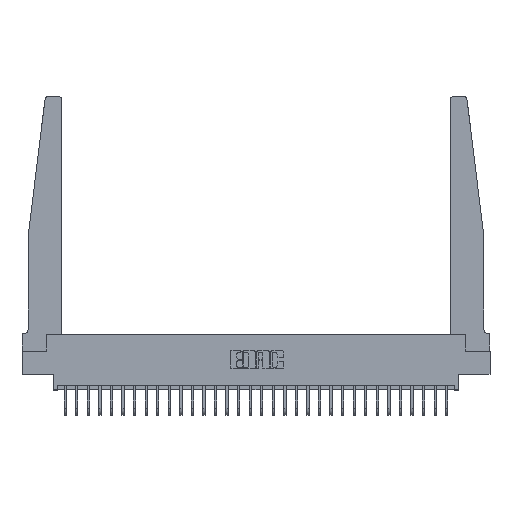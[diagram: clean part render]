
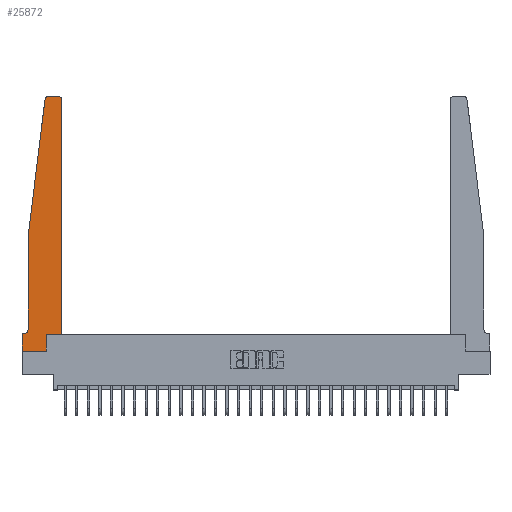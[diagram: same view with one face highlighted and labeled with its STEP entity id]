
A CAD part, top view. The second image highlights one B-rep face of the part: STEP entity #25872.
In plain terms, the highlighted planar face has unit normal (0, 0, 1).
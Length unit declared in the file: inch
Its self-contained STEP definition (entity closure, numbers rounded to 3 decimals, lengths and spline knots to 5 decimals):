
#202 = EDGE_CURVE ( 'NONE', #3517, #4428, #2858, .T. ) ;
#236 = AXIS2_PLACEMENT_3D ( 'NONE', #23653, #11117, #25749 ) ;
#385 = LINE ( 'NONE', #25950, #16533 ) ;
#737 = PLANE ( 'NONE',  #3675 ) ;
#984 = VERTEX_POINT ( 'NONE', #1517 ) ;
#1458 = EDGE_CURVE ( 'NONE', #24865, #11048, #17905, .T. ) ;
#1476 = ORIENTED_EDGE ( 'NONE', *, *, #18724, .T. ) ;
#1517 = CARTESIAN_POINT ( 'NONE',  ( 0.395, 2.75, 0.37 ) ) ;
#1602 = CARTESIAN_POINT ( 'NONE',  ( 0., 0., 0.37 ) ) ;
#1694 = ORIENTED_EDGE ( 'NONE', *, *, #8246, .T. ) ;
#2197 = VECTOR ( 'NONE', #7533, 39.37008 ) ;
#2371 = DIRECTION ( 'NONE',  ( 1., 0., 0. ) ) ;
#2480 = LINE ( 'NONE', #26995, #14278 ) ;
#2668 = CARTESIAN_POINT ( 'NONE',  ( 0.065, 1.25, 0.37 ) ) ;
#2858 = LINE ( 'NONE', #16054, #2197 ) ;
#3030 = VERTEX_POINT ( 'NONE', #4614 ) ;
#3064 = CARTESIAN_POINT ( 'NONE',  ( 0.27653, 2.75, 0.37 ) ) ;
#3068 = ORIENTED_EDGE ( 'NONE', *, *, #202, .T. ) ;
#3286 = CARTESIAN_POINT ( 'NONE',  ( 0.065, 1.25, 0.37 ) ) ;
#3517 = VERTEX_POINT ( 'NONE', #15203 ) ;
#3675 = AXIS2_PLACEMENT_3D ( 'NONE', #17577, #5014, #19673 ) ;
#3936 = EDGE_CURVE ( 'NONE', #25004, #24865, #8726, .T. ) ;
#4331 = VECTOR ( 'NONE', #26123, 39.37008 ) ;
#4428 = VERTEX_POINT ( 'NONE', #3286 ) ;
#4562 = DIRECTION ( 'NONE',  ( 0., 0., 1. ) ) ;
#4614 = CARTESIAN_POINT ( 'NONE',  ( 0.015, 0.1875, 0.37 ) ) ;
#4989 = EDGE_LOOP ( 'NONE', ( #1694, #9234, #3068, #1476, #12937, #21291, #25565, #26475, #20586, #14266, #13524, #8286 ) ) ;
#5014 = DIRECTION ( 'NONE',  ( 0., 0., 1. ) ) ;
#5587 = CARTESIAN_POINT ( 'NONE',  ( 0.2605, 0., 0.37 ) ) ;
#5908 = CARTESIAN_POINT ( 'NONE',  ( 0.015, 0.2375, 0.37 ) ) ;
#6097 = AXIS2_PLACEMENT_3D ( 'NONE', #17130, #4562, #19234 ) ;
#6887 = VERTEX_POINT ( 'NONE', #3064 ) ;
#6914 = EDGE_CURVE ( 'NONE', #13854, #25004, #7936, .T. ) ;
#7533 = DIRECTION ( 'NONE',  ( -0.122, -0.992, 0. ) ) ;
#7851 = AXIS2_PLACEMENT_3D ( 'NONE', #5908, #20555, #8011 ) ;
#7936 = LINE ( 'NONE', #11473, #4331 ) ;
#8011 = DIRECTION ( 'NONE',  ( -1., 0., 0. ) ) ;
#8246 = EDGE_CURVE ( 'NONE', #984, #6887, #25530, .T. ) ;
#8286 = ORIENTED_EDGE ( 'NONE', *, *, #12758, .T. ) ;
#8726 = LINE ( 'NONE', #17132, #19227 ) ;
#8829 = VECTOR ( 'NONE', #17255, 39.37008 ) ;
#9234 = ORIENTED_EDGE ( 'NONE', *, *, #12041, .T. ) ;
#10289 = CARTESIAN_POINT ( 'NONE',  ( 0.2605, 0.18, 0.37 ) ) ;
#10714 = CIRCLE ( 'NONE', #236, 0.03 ) ;
#10925 = CARTESIAN_POINT ( 'NONE',  ( 0.25, 2.75, 0.37 ) ) ;
#11048 = VERTEX_POINT ( 'NONE', #17717 ) ;
#11117 = DIRECTION ( 'NONE',  ( 0., 0., 1. ) ) ;
#11409 = DIRECTION ( 'NONE',  ( 0., 1., 0. ) ) ;
#11413 = VERTEX_POINT ( 'NONE', #12524 ) ;
#11473 = CARTESIAN_POINT ( 'NONE',  ( 0.2605, 0.18, 0.37 ) ) ;
#11853 = VERTEX_POINT ( 'NONE', #1602 ) ;
#12041 = EDGE_CURVE ( 'NONE', #6887, #3517, #22228, .T. ) ;
#12279 = VECTOR ( 'NONE', #11409, 39.37008 ) ;
#12524 = CARTESIAN_POINT ( 'NONE',  ( 0.065, 0.2375, 0.37 ) ) ;
#12758 = EDGE_CURVE ( 'NONE', #11048, #984, #10714, .T. ) ;
#12851 = VECTOR ( 'NONE', #2371, 39.37008 ) ;
#12937 = ORIENTED_EDGE ( 'NONE', *, *, #24080, .T. ) ;
#13348 = EDGE_CURVE ( 'NONE', #21468, #11853, #2480, .T. ) ;
#13512 = LINE ( 'NONE', #17061, #12851 ) ;
#13524 = ORIENTED_EDGE ( 'NONE', *, *, #1458, .T. ) ;
#13854 = VERTEX_POINT ( 'NONE', #5587 ) ;
#14266 = ORIENTED_EDGE ( 'NONE', *, *, #3936, .T. ) ;
#14278 = VECTOR ( 'NONE', #14477, 39.37008 ) ;
#14477 = DIRECTION ( 'NONE',  ( 0., -1., 0. ) ) ;
#14757 = VECTOR ( 'NONE', #17362, 39.37008 ) ;
#15203 = CARTESIAN_POINT ( 'NONE',  ( 0.24675, 2.72367, 0.37 ) ) ;
#15535 = CARTESIAN_POINT ( 'NONE',  ( 0.425, 0.18, 0.37 ) ) ;
#15771 = CIRCLE ( 'NONE', #7851, 0.05 ) ;
#15826 = CARTESIAN_POINT ( 'NONE',  ( 0., 0.1875, 0.37 ) ) ;
#16054 = CARTESIAN_POINT ( 'NONE',  ( 0.065, 1.25, 0.37 ) ) ;
#16533 = VECTOR ( 'NONE', #23948, 39.37008 ) ;
#17049 = EDGE_CURVE ( 'NONE', #3030, #21468, #385, .T. ) ;
#17061 = CARTESIAN_POINT ( 'NONE',  ( 0., 0., 0.37 ) ) ;
#17130 = CARTESIAN_POINT ( 'NONE',  ( 0.27653, 2.72, 0.37 ) ) ;
#17132 = CARTESIAN_POINT ( 'NONE',  ( 0.425, 0.18, 0.37 ) ) ;
#17255 = DIRECTION ( 'NONE',  ( -1., 0., 0. ) ) ;
#17362 = DIRECTION ( 'NONE',  ( 0., -1., 0. ) ) ;
#17577 = CARTESIAN_POINT ( 'NONE',  ( 0., 0.1875, 0.37 ) ) ;
#17717 = CARTESIAN_POINT ( 'NONE',  ( 0.425, 2.72, 0.37 ) ) ;
#17905 = LINE ( 'NONE', #15535, #12279 ) ;
#18724 = EDGE_CURVE ( 'NONE', #4428, #11413, #20345, .T. ) ;
#19153 = DIRECTION ( 'NONE',  ( 1., 0., 0. ) ) ;
#19227 = VECTOR ( 'NONE', #19153, 39.37008 ) ;
#19234 = DIRECTION ( 'NONE',  ( 1., 0., 0. ) ) ;
#19673 = DIRECTION ( 'NONE',  ( 1., 0., 0. ) ) ;
#20345 = LINE ( 'NONE', #2668, #14757 ) ;
#20555 = DIRECTION ( 'NONE',  ( 0., 0., -1. ) ) ;
#20583 = FACE_OUTER_BOUND ( 'NONE', #4989, .T. ) ;
#20586 = ORIENTED_EDGE ( 'NONE', *, *, #6914, .T. ) ;
#21291 = ORIENTED_EDGE ( 'NONE', *, *, #17049, .T. ) ;
#21468 = VERTEX_POINT ( 'NONE', #15826 ) ;
#22228 = CIRCLE ( 'NONE', #6097, 0.03 ) ;
#22974 = EDGE_CURVE ( 'NONE', #11853, #13854, #13512, .T. ) ;
#23653 = CARTESIAN_POINT ( 'NONE',  ( 0.395, 2.72, 0.37 ) ) ;
#23948 = DIRECTION ( 'NONE',  ( -1., 0., 0. ) ) ;
#24080 = EDGE_CURVE ( 'NONE', #11413, #3030, #15771, .T. ) ;
#24458 = CARTESIAN_POINT ( 'NONE',  ( 0.425, 0.18, 0.37 ) ) ;
#24865 = VERTEX_POINT ( 'NONE', #24458 ) ;
#25004 = VERTEX_POINT ( 'NONE', #10289 ) ;
#25530 = LINE ( 'NONE', #10925, #8829 ) ;
#25565 = ORIENTED_EDGE ( 'NONE', *, *, #13348, .T. ) ;
#25749 = DIRECTION ( 'NONE',  ( 1., 0., 0. ) ) ;
#25872 = ADVANCED_FACE ( 'NONE', ( #20583 ), #737, .T. ) ;
#25950 = CARTESIAN_POINT ( 'NONE',  ( 0.065, 0.1875, 0.37 ) ) ;
#26123 = DIRECTION ( 'NONE',  ( 0., 1., 0. ) ) ;
#26475 = ORIENTED_EDGE ( 'NONE', *, *, #22974, .T. ) ;
#26995 = CARTESIAN_POINT ( 'NONE',  ( 0., 0., 0.37 ) ) ;
